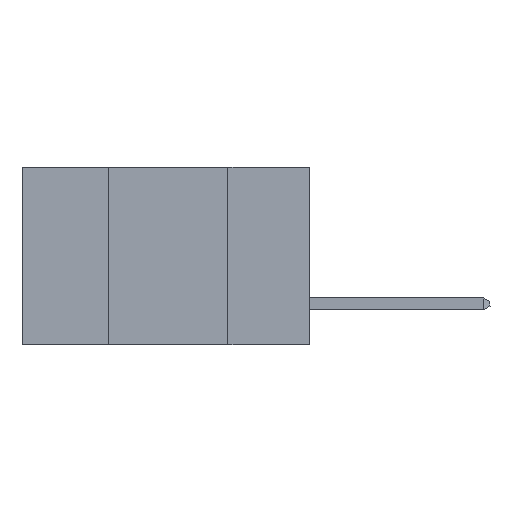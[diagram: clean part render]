
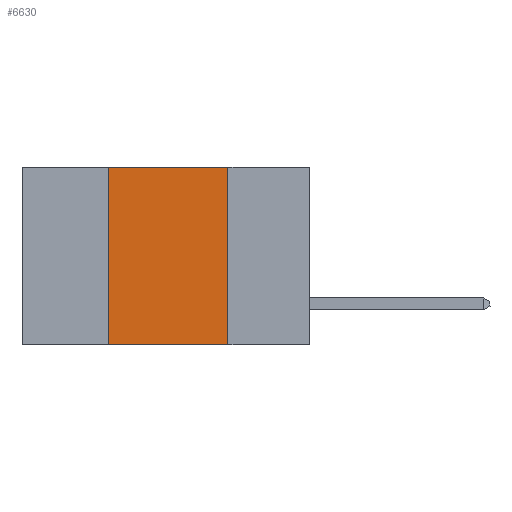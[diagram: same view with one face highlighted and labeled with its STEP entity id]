
A CAD part, left-side view. The second image highlights one B-rep face of the part: STEP entity #6630.
In plain terms, the highlighted planar face has unit normal (-1, 0, 0).
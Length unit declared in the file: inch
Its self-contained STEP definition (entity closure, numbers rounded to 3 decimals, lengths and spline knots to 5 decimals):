
#27 = DIRECTION ( 'NONE',  ( 0., -1., 0. ) ) ;
#236 = LINE ( 'NONE', #12593, #14051 ) ;
#511 = CARTESIAN_POINT ( 'NONE',  ( 0., 0.17, 0. ) ) ;
#1272 = VERTEX_POINT ( 'NONE', #3817 ) ;
#1818 = DIRECTION ( 'NONE',  ( 0., 0., 1. ) ) ;
#2320 = EDGE_CURVE ( 'NONE', #8214, #1272, #4902, .T. ) ;
#2425 = VECTOR ( 'NONE', #27, 39.37008 ) ;
#2657 = DIRECTION ( 'NONE',  ( 0., 0., -1. ) ) ;
#2872 = CARTESIAN_POINT ( 'NONE',  ( 0., 0.42, 0. ) ) ;
#3401 = DIRECTION ( 'NONE',  ( 0., -1., 0. ) ) ;
#3817 = CARTESIAN_POINT ( 'NONE',  ( 0., 0.42, 0. ) ) ;
#4356 = ORIENTED_EDGE ( 'NONE', *, *, #2320, .F. ) ;
#4860 = DIRECTION ( 'NONE',  ( 1., 0., 0. ) ) ;
#4902 = LINE ( 'NONE', #2872, #12324 ) ;
#4955 = CARTESIAN_POINT ( 'NONE',  ( 0., 0.42, -0.37 ) ) ;
#5059 = CARTESIAN_POINT ( 'NONE',  ( 0., 0.6, 0. ) ) ;
#5505 = LINE ( 'NONE', #7974, #2425 ) ;
#5790 = CARTESIAN_POINT ( 'NONE',  ( 0., 0.17, 0. ) ) ;
#5850 = ORIENTED_EDGE ( 'NONE', *, *, #7111, .T. ) ;
#6157 = PLANE ( 'NONE',  #8852 ) ;
#6360 = ORIENTED_EDGE ( 'NONE', *, *, #12294, .F. ) ;
#6630 = ADVANCED_FACE ( 'NONE', ( #10595 ), #6157, .F. ) ;
#7111 = EDGE_CURVE ( 'NONE', #8214, #8523, #5505, .T. ) ;
#7631 = LINE ( 'NONE', #5790, #11441 ) ;
#7974 = CARTESIAN_POINT ( 'NONE',  ( 0., 0.6, -0.37 ) ) ;
#8214 = VERTEX_POINT ( 'NONE', #4955 ) ;
#8523 = VERTEX_POINT ( 'NONE', #11411 ) ;
#8852 = AXIS2_PLACEMENT_3D ( 'NONE', #5059, #4860, #2657 ) ;
#10595 = FACE_OUTER_BOUND ( 'NONE', #14252, .T. ) ;
#11411 = CARTESIAN_POINT ( 'NONE',  ( 0., 0.17, -0.37 ) ) ;
#11441 = VECTOR ( 'NONE', #12698, 39.37008 ) ;
#12088 = ORIENTED_EDGE ( 'NONE', *, *, #14125, .F. ) ;
#12294 = EDGE_CURVE ( 'NONE', #1272, #12898, #236, .T. ) ;
#12324 = VECTOR ( 'NONE', #1818, 39.37008 ) ;
#12593 = CARTESIAN_POINT ( 'NONE',  ( 0., 0.6, 0. ) ) ;
#12698 = DIRECTION ( 'NONE',  ( 0., 0., -1. ) ) ;
#12898 = VERTEX_POINT ( 'NONE', #511 ) ;
#14051 = VECTOR ( 'NONE', #3401, 39.37008 ) ;
#14125 = EDGE_CURVE ( 'NONE', #12898, #8523, #7631, .T. ) ;
#14252 = EDGE_LOOP ( 'NONE', ( #12088, #6360, #4356, #5850 ) ) ;
